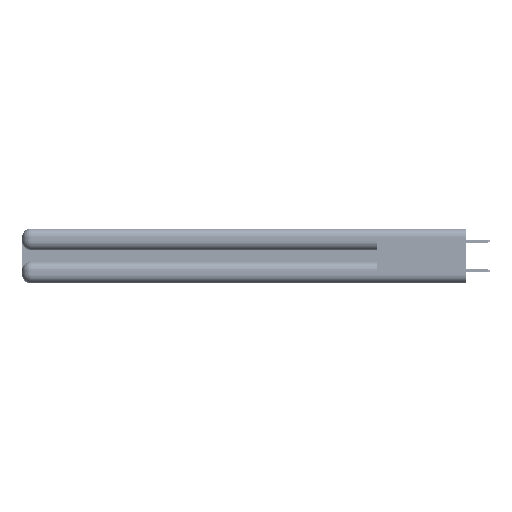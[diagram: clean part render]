
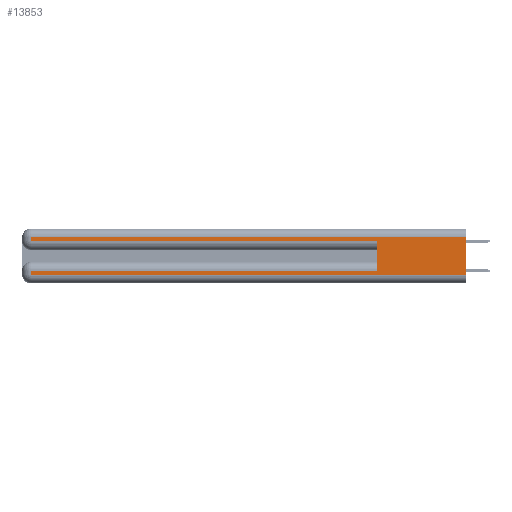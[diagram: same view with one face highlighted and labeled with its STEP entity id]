
A CAD part, left-side view. The second image highlights one B-rep face of the part: STEP entity #13853.
In plain terms, the highlighted planar face has unit normal (-1, 0, 0).
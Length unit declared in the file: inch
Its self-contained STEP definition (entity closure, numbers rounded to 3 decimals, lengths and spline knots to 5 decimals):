
#25 = LINE ( 'NONE', #32904, #8815 ) ;
#254 = ORIENTED_EDGE ( 'NONE', *, *, #35137, .F. ) ;
#621 = ORIENTED_EDGE ( 'NONE', *, *, #12108, .T. ) ;
#1175 = AXIS2_PLACEMENT_3D ( 'NONE', #18267, #48423, #22625 ) ;
#2222 = VERTEX_POINT ( 'NONE', #5669 ) ;
#2629 = DIRECTION ( 'NONE',  ( 0., -1., 0. ) ) ;
#3007 = VERTEX_POINT ( 'NONE', #40640 ) ;
#3947 = EDGE_CURVE ( 'NONE', #29386, #8733, #25274, .T. ) ;
#5669 = CARTESIAN_POINT ( 'NONE',  ( 0., 2.94, 0.31 ) ) ;
#6430 = CARTESIAN_POINT ( 'NONE',  ( 0., 0., 0.37 ) ) ;
#6481 = ORIENTED_EDGE ( 'NONE', *, *, #37626, .T. ) ;
#6527 = EDGE_CURVE ( 'NONE', #30232, #3007, #25, .T. ) ;
#8067 = VECTOR ( 'NONE', #16025, 39.37008 ) ;
#8733 = VERTEX_POINT ( 'NONE', #18827 ) ;
#8815 = VECTOR ( 'NONE', #45926, 39.37008 ) ;
#10756 = DIRECTION ( 'NONE',  ( 0., 0., -1. ) ) ;
#11508 = VECTOR ( 'NONE', #10756, 39.37008 ) ;
#12108 = EDGE_CURVE ( 'NONE', #2222, #29386, #25863, .T. ) ;
#12437 = ORIENTED_EDGE ( 'NONE', *, *, #19378, .T. ) ;
#13643 = ORIENTED_EDGE ( 'NONE', *, *, #24358, .T. ) ;
#13853 = ADVANCED_FACE ( 'NONE', ( #51254 ), #13944, .F. ) ;
#13944 = PLANE ( 'NONE',  #1175 ) ;
#14027 = EDGE_CURVE ( 'NONE', #51990, #50358, #31731, .T. ) ;
#16025 = DIRECTION ( 'NONE',  ( 0., 0., 1. ) ) ;
#16401 = CARTESIAN_POINT ( 'NONE',  ( 0., 0., 0.31 ) ) ;
#16671 = DIRECTION ( 'NONE',  ( 0., 0., -1. ) ) ;
#16974 = EDGE_LOOP ( 'NONE', ( #36266, #6481, #621, #54603, #254, #12437, #32014, #13643 ) ) ;
#17098 = CARTESIAN_POINT ( 'NONE',  ( 0., 0., 0.31 ) ) ;
#17827 = CARTESIAN_POINT ( 'NONE',  ( 0., 2.94, 0.085 ) ) ;
#18267 = CARTESIAN_POINT ( 'NONE',  ( 0., 0., 0.37 ) ) ;
#18482 = DIRECTION ( 'NONE',  ( 0., -1., 0. ) ) ;
#18827 = CARTESIAN_POINT ( 'NONE',  ( 0., 0.6, 0.285 ) ) ;
#19378 = EDGE_CURVE ( 'NONE', #19716, #30232, #42863, .T. ) ;
#19716 = VERTEX_POINT ( 'NONE', #39947 ) ;
#22625 = DIRECTION ( 'NONE',  ( 0., 0., -1. ) ) ;
#24088 = CARTESIAN_POINT ( 'NONE',  ( 0., 0., 0.06 ) ) ;
#24358 = EDGE_CURVE ( 'NONE', #3007, #50358, #33796, .T. ) ;
#25274 = LINE ( 'NONE', #30166, #35389 ) ;
#25863 = LINE ( 'NONE', #42502, #48802 ) ;
#29053 = CARTESIAN_POINT ( 'NONE',  ( 0., 0.6, 0.145 ) ) ;
#29386 = VERTEX_POINT ( 'NONE', #55561 ) ;
#30166 = CARTESIAN_POINT ( 'NONE',  ( 0., 0., 0.285 ) ) ;
#30232 = VERTEX_POINT ( 'NONE', #17827 ) ;
#31335 = VECTOR ( 'NONE', #46574, 39.37008 ) ;
#31731 = LINE ( 'NONE', #6430, #11508 ) ;
#32014 = ORIENTED_EDGE ( 'NONE', *, *, #6527, .T. ) ;
#32348 = LINE ( 'NONE', #29053, #8067 ) ;
#32904 = CARTESIAN_POINT ( 'NONE',  ( 0., 2.94, 0.37 ) ) ;
#33796 = LINE ( 'NONE', #24088, #55338 ) ;
#34105 = DIRECTION ( 'NONE',  ( 0., 1., 0. ) ) ;
#35137 = EDGE_CURVE ( 'NONE', #19716, #8733, #32348, .T. ) ;
#35389 = VECTOR ( 'NONE', #18482, 39.37008 ) ;
#36266 = ORIENTED_EDGE ( 'NONE', *, *, #14027, .F. ) ;
#37626 = EDGE_CURVE ( 'NONE', #51990, #2222, #42792, .T. ) ;
#39947 = CARTESIAN_POINT ( 'NONE',  ( 0., 0.6, 0.085 ) ) ;
#40640 = CARTESIAN_POINT ( 'NONE',  ( 0., 2.94, 0.06 ) ) ;
#41537 = VECTOR ( 'NONE', #34105, 39.37008 ) ;
#42502 = CARTESIAN_POINT ( 'NONE',  ( 0., 2.94, 0.37 ) ) ;
#42792 = LINE ( 'NONE', #16401, #31335 ) ;
#42863 = LINE ( 'NONE', #46941, #41537 ) ;
#45926 = DIRECTION ( 'NONE',  ( 0., 0., -1. ) ) ;
#46574 = DIRECTION ( 'NONE',  ( 0., 1., 0. ) ) ;
#46941 = CARTESIAN_POINT ( 'NONE',  ( 0., 0., 0.085 ) ) ;
#48423 = DIRECTION ( 'NONE',  ( 1., 0., 0. ) ) ;
#48802 = VECTOR ( 'NONE', #16671, 39.37008 ) ;
#50358 = VERTEX_POINT ( 'NONE', #52775 ) ;
#51254 = FACE_OUTER_BOUND ( 'NONE', #16974, .T. ) ;
#51990 = VERTEX_POINT ( 'NONE', #17098 ) ;
#52775 = CARTESIAN_POINT ( 'NONE',  ( 0., 0., 0.06 ) ) ;
#54603 = ORIENTED_EDGE ( 'NONE', *, *, #3947, .T. ) ;
#55338 = VECTOR ( 'NONE', #2629, 39.37008 ) ;
#55561 = CARTESIAN_POINT ( 'NONE',  ( 0., 2.94, 0.285 ) ) ;
